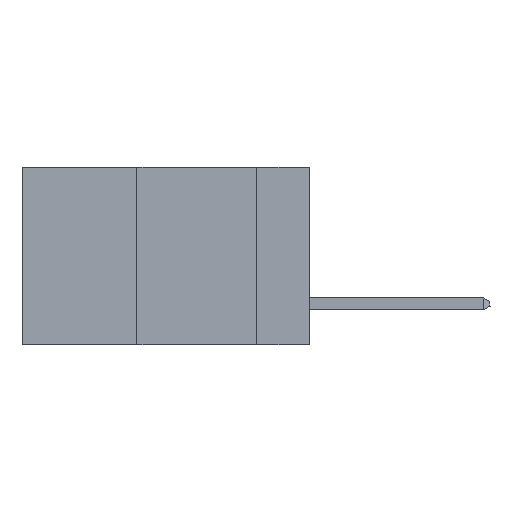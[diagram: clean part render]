
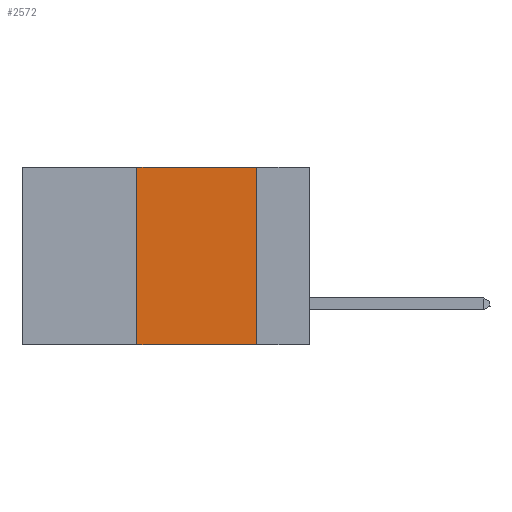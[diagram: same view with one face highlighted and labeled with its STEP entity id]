
A CAD part, left-side view. The second image highlights one B-rep face of the part: STEP entity #2572.
In plain terms, the highlighted planar face has unit normal (-1, 0, 0).
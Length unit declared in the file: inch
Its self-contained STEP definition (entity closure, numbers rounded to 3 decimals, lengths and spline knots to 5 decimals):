
#2065 = CARTESIAN_POINT ( 'NONE',  ( 0., 0.6, 0. ) ) ;
#2273 = LINE ( 'NONE', #6645, #21662 ) ;
#2572 = ADVANCED_FACE ( 'NONE', ( #9342 ), #14698, .F. ) ;
#6317 = VERTEX_POINT ( 'NONE', #25286 ) ;
#6645 = CARTESIAN_POINT ( 'NONE',  ( 0., 0.11, 0. ) ) ;
#7128 = DIRECTION ( 'NONE',  ( 0., -1., 0. ) ) ;
#9342 = FACE_OUTER_BOUND ( 'NONE', #16997, .T. ) ;
#9770 = VECTOR ( 'NONE', #10922, 39.37008 ) ;
#9847 = DIRECTION ( 'NONE',  ( 0., 0., -1. ) ) ;
#10829 = AXIS2_PLACEMENT_3D ( 'NONE', #2065, #30365, #18075 ) ;
#10922 = DIRECTION ( 'NONE',  ( 0., -1., 0. ) ) ;
#12591 = DIRECTION ( 'NONE',  ( 0., 0., 1. ) ) ;
#14698 = PLANE ( 'NONE',  #10829 ) ;
#16260 = LINE ( 'NONE', #31235, #9770 ) ;
#16997 = EDGE_LOOP ( 'NONE', ( #40390, #20500, #22898, #17458 ) ) ;
#17458 = ORIENTED_EDGE ( 'NONE', *, *, #22077, .T. ) ;
#17700 = CARTESIAN_POINT ( 'NONE',  ( 0., 0.11, -0.37 ) ) ;
#18075 = DIRECTION ( 'NONE',  ( 0., 0., -1. ) ) ;
#18294 = EDGE_CURVE ( 'NONE', #6317, #40369, #16260, .T. ) ;
#19412 = VERTEX_POINT ( 'NONE', #31296 ) ;
#20500 = ORIENTED_EDGE ( 'NONE', *, *, #18294, .F. ) ;
#20802 = VECTOR ( 'NONE', #12591, 39.37008 ) ;
#21442 = VERTEX_POINT ( 'NONE', #17700 ) ;
#21662 = VECTOR ( 'NONE', #9847, 39.37008 ) ;
#22077 = EDGE_CURVE ( 'NONE', #19412, #21442, #32488, .T. ) ;
#22898 = ORIENTED_EDGE ( 'NONE', *, *, #26316, .F. ) ;
#25286 = CARTESIAN_POINT ( 'NONE',  ( 0., 0.36, 0. ) ) ;
#26316 = EDGE_CURVE ( 'NONE', #19412, #6317, #27754, .T. ) ;
#27754 = LINE ( 'NONE', #38416, #20802 ) ;
#30365 = DIRECTION ( 'NONE',  ( 1., 0., 0. ) ) ;
#31235 = CARTESIAN_POINT ( 'NONE',  ( 0., 0.6, 0. ) ) ;
#31296 = CARTESIAN_POINT ( 'NONE',  ( 0., 0.36, -0.37 ) ) ;
#32488 = LINE ( 'NONE', #32894, #38431 ) ;
#32894 = CARTESIAN_POINT ( 'NONE',  ( 0., 0.6, -0.37 ) ) ;
#38416 = CARTESIAN_POINT ( 'NONE',  ( 0., 0.36, 0. ) ) ;
#38431 = VECTOR ( 'NONE', #7128, 39.37008 ) ;
#39905 = CARTESIAN_POINT ( 'NONE',  ( 0., 0.11, 0. ) ) ;
#40369 = VERTEX_POINT ( 'NONE', #39905 ) ;
#40390 = ORIENTED_EDGE ( 'NONE', *, *, #40489, .F. ) ;
#40489 = EDGE_CURVE ( 'NONE', #40369, #21442, #2273, .T. ) ;
